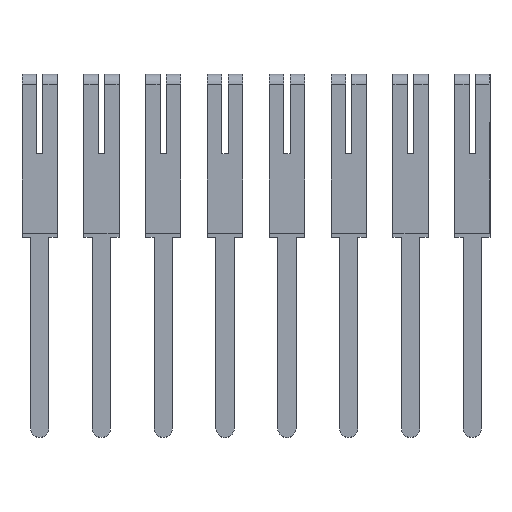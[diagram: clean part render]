
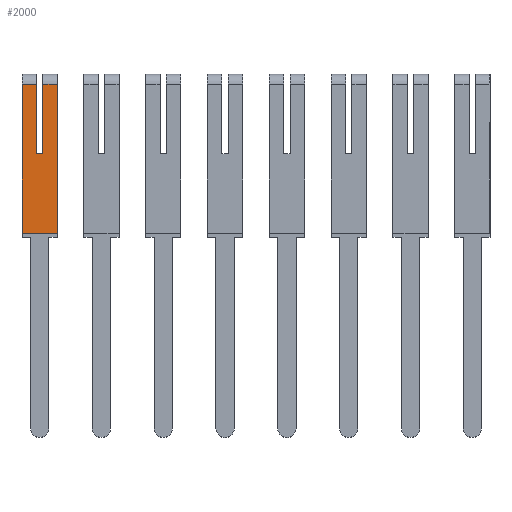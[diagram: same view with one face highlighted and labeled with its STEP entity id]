
A CAD part, top view. The second image highlights one B-rep face of the part: STEP entity #2000.
In plain terms, the highlighted face is planar.
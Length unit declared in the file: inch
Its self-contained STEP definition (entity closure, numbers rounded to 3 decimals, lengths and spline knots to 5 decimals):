
#168 = EDGE_CURVE ( 'NONE', #9361, #8459, #3602, .T. ) ;
#239 = ORIENTED_EDGE ( 'NONE', *, *, #3464, .F. ) ;
#383 = DIRECTION ( 'NONE',  ( 0., 1., 0. ) ) ;
#548 = ORIENTED_EDGE ( 'NONE', *, *, #3300, .T. ) ;
#602 = ORIENTED_EDGE ( 'NONE', *, *, #3481, .F. ) ;
#1071 = EDGE_LOOP ( 'NONE', ( #548, #9442, #2717, #239, #5454, #4508, #602, #4542 ) ) ;
#1185 = CARTESIAN_POINT ( 'NONE',  ( 0.215, 0.27975, -0.0365 ) ) ;
#1308 = VECTOR ( 'NONE', #6843, 39.37008 ) ;
#1357 = LINE ( 'NONE', #9201, #4313 ) ;
#1651 = LINE ( 'NONE', #8177, #7180 ) ;
#1999 = DIRECTION ( 'NONE',  ( 0., 1., 0. ) ) ;
#2000 = ADVANCED_FACE ( 'NONE', ( #9413 ), #6166, .T. ) ;
#2206 = CARTESIAN_POINT ( 'NONE',  ( 0.215, 0., -0.089 ) ) ;
#2717 = ORIENTED_EDGE ( 'NONE', *, *, #3386, .F. ) ;
#3282 = EDGE_CURVE ( 'NONE', #5534, #4946, #1357, .T. ) ;
#3300 = EDGE_CURVE ( 'NONE', #3361, #5534, #11815, .T. ) ;
#3344 = CARTESIAN_POINT ( 'NONE',  ( 0.215, 0., 0. ) ) ;
#3361 = VERTEX_POINT ( 'NONE', #5371 ) ;
#3386 = EDGE_CURVE ( 'NONE', #7623, #4946, #9899, .T. ) ;
#3464 = EDGE_CURVE ( 'NONE', #8764, #7623, #1651, .T. ) ;
#3467 = EDGE_CURVE ( 'NONE', #8764, #9361, #4603, .T. ) ;
#3481 = EDGE_CURVE ( 'NONE', #7852, #8459, #11104, .T. ) ;
#3485 = EDGE_CURVE ( 'NONE', #3361, #7852, #6624, .T. ) ;
#3602 = LINE ( 'NONE', #10767, #8680 ) ;
#3935 = VECTOR ( 'NONE', #1999, 39.37008 ) ;
#4313 = VECTOR ( 'NONE', #4816, 39.37008 ) ;
#4508 = ORIENTED_EDGE ( 'NONE', *, *, #168, .T. ) ;
#4542 = ORIENTED_EDGE ( 'NONE', *, *, #3485, .F. ) ;
#4566 = DIRECTION ( 'NONE',  ( 0., 1., 0. ) ) ;
#4603 = LINE ( 'NONE', #2206, #1308 ) ;
#4734 = CARTESIAN_POINT ( 'NONE',  ( 0.215, -0.096, 0. ) ) ;
#4816 = DIRECTION ( 'NONE',  ( 0., 0., 1. ) ) ;
#4946 = VERTEX_POINT ( 'NONE', #10433 ) ;
#5371 = CARTESIAN_POINT ( 'NONE',  ( 0.215, 0.105, -0.0365 ) ) ;
#5454 = ORIENTED_EDGE ( 'NONE', *, *, #3467, .T. ) ;
#5534 = VERTEX_POINT ( 'NONE', #1185 ) ;
#5598 = CARTESIAN_POINT ( 'NONE',  ( 0.215, 0.27975, -0.0525 ) ) ;
#6159 = DIRECTION ( 'NONE',  ( 1., 0., 0. ) ) ;
#6166 = PLANE ( 'NONE',  #8337 ) ;
#6624 = LINE ( 'NONE', #9217, #10857 ) ;
#6823 = CARTESIAN_POINT ( 'NONE',  ( 0.215, 0.105, -0.0525 ) ) ;
#6843 = DIRECTION ( 'NONE',  ( 0., 1., 0. ) ) ;
#6862 = CARTESIAN_POINT ( 'NONE',  ( 0.215, -0.096, -0.089 ) ) ;
#7180 = VECTOR ( 'NONE', #9928, 39.37008 ) ;
#7623 = VERTEX_POINT ( 'NONE', #4734 ) ;
#7852 = VERTEX_POINT ( 'NONE', #6823 ) ;
#8167 = CARTESIAN_POINT ( 'NONE',  ( 0.215, 0.27975, -0.089 ) ) ;
#8177 = CARTESIAN_POINT ( 'NONE',  ( 0.215, -0.096, -0.089 ) ) ;
#8317 = CARTESIAN_POINT ( 'NONE',  ( 0.215, 0.105, -0.0365 ) ) ;
#8337 = AXIS2_PLACEMENT_3D ( 'NONE', #10827, #6159, #383 ) ;
#8459 = VERTEX_POINT ( 'NONE', #5598 ) ;
#8680 = VECTOR ( 'NONE', #10374, 39.37008 ) ;
#8764 = VERTEX_POINT ( 'NONE', #6862 ) ;
#9201 = CARTESIAN_POINT ( 'NONE',  ( 0.215, 0.27975, -0.089 ) ) ;
#9217 = CARTESIAN_POINT ( 'NONE',  ( 0.215, 0.105, -0.0365 ) ) ;
#9361 = VERTEX_POINT ( 'NONE', #8167 ) ;
#9413 = FACE_OUTER_BOUND ( 'NONE', #1071, .T. ) ;
#9442 = ORIENTED_EDGE ( 'NONE', *, *, #3282, .T. ) ;
#9480 = DIRECTION ( 'NONE',  ( 0., 1., 0. ) ) ;
#9899 = LINE ( 'NONE', #3344, #11700 ) ;
#9928 = DIRECTION ( 'NONE',  ( 0., 0., 1. ) ) ;
#10374 = DIRECTION ( 'NONE',  ( 0., 0., 1. ) ) ;
#10433 = CARTESIAN_POINT ( 'NONE',  ( 0.215, 0.27975, 0. ) ) ;
#10767 = CARTESIAN_POINT ( 'NONE',  ( 0.215, 0.27975, -0.089 ) ) ;
#10827 = CARTESIAN_POINT ( 'NONE',  ( 0.215, 0., -0.089 ) ) ;
#10857 = VECTOR ( 'NONE', #11827, 39.37008 ) ;
#10889 = VECTOR ( 'NONE', #4566, 39.37008 ) ;
#11104 = LINE ( 'NONE', #12184, #3935 ) ;
#11700 = VECTOR ( 'NONE', #9480, 39.37008 ) ;
#11815 = LINE ( 'NONE', #8317, #10889 ) ;
#11827 = DIRECTION ( 'NONE',  ( 0., 0., -1. ) ) ;
#12184 = CARTESIAN_POINT ( 'NONE',  ( 0.215, 0.105, -0.0525 ) ) ;
